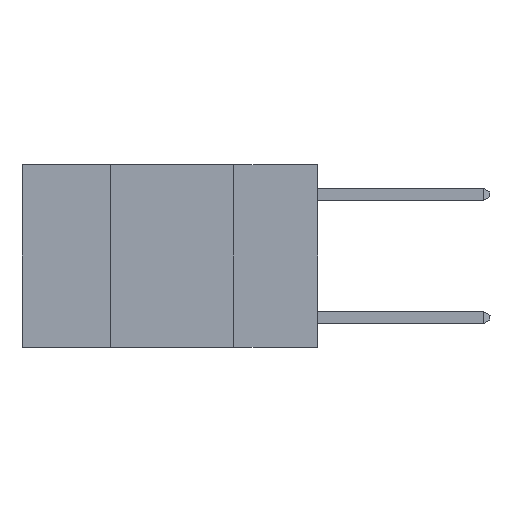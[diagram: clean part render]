
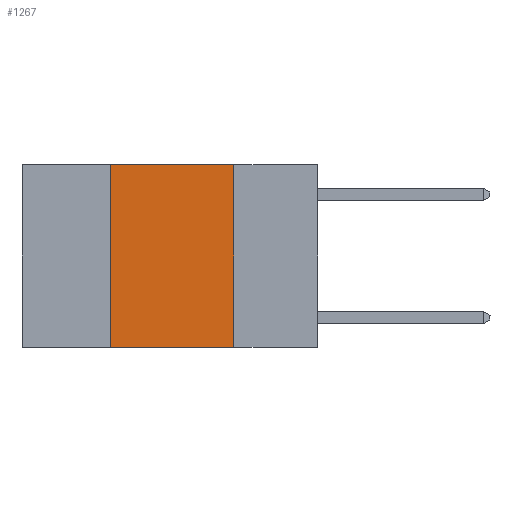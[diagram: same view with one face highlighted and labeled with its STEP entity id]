
A CAD part, left-side view. The second image highlights one B-rep face of the part: STEP entity #1267.
In plain terms, the highlighted planar face has unit normal (-1, 0, 0).
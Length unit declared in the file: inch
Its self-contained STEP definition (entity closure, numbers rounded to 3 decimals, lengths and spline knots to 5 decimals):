
#1013 = EDGE_CURVE ( 'NONE', #4432, #13708, #11321, .T. ) ;
#1029 = CARTESIAN_POINT ( 'NONE',  ( 0., 0.42, 0. ) ) ;
#1267 = ADVANCED_FACE ( 'NONE', ( #11890 ), #11979, .F. ) ;
#1552 = CARTESIAN_POINT ( 'NONE',  ( 0., 0.17, 0. ) ) ;
#1984 = VERTEX_POINT ( 'NONE', #16516 ) ;
#2218 = DIRECTION ( 'NONE',  ( 0., 0., 1. ) ) ;
#2761 = EDGE_CURVE ( 'NONE', #1984, #17518, #3835, .T. ) ;
#3797 = EDGE_CURVE ( 'NONE', #13708, #17518, #4165, .T. ) ;
#3835 = LINE ( 'NONE', #9848, #17311 ) ;
#4017 = CARTESIAN_POINT ( 'NONE',  ( 0., 0.6, 0. ) ) ;
#4165 = LINE ( 'NONE', #1552, #17338 ) ;
#4432 = VERTEX_POINT ( 'NONE', #6509 ) ;
#4508 = VECTOR ( 'NONE', #14210, 39.37008 ) ;
#5514 = EDGE_CURVE ( 'NONE', #1984, #4432, #8598, .T. ) ;
#6509 = CARTESIAN_POINT ( 'NONE',  ( 0., 0.42, 0. ) ) ;
#7921 = CARTESIAN_POINT ( 'NONE',  ( 0., 0.17, 0. ) ) ;
#8598 = LINE ( 'NONE', #1029, #18716 ) ;
#8946 = ORIENTED_EDGE ( 'NONE', *, *, #2761, .T. ) ;
#9848 = CARTESIAN_POINT ( 'NONE',  ( 0., 0.6, -0.37 ) ) ;
#10430 = DIRECTION ( 'NONE',  ( 0., 0., -1. ) ) ;
#11273 = ORIENTED_EDGE ( 'NONE', *, *, #5514, .F. ) ;
#11321 = LINE ( 'NONE', #4017, #4508 ) ;
#11365 = CARTESIAN_POINT ( 'NONE',  ( 0., 0.17, -0.37 ) ) ;
#11433 = AXIS2_PLACEMENT_3D ( 'NONE', #14890, #17794, #10430 ) ;
#11519 = DIRECTION ( 'NONE',  ( 0., -1., 0. ) ) ;
#11890 = FACE_OUTER_BOUND ( 'NONE', #14209, .T. ) ;
#11979 = PLANE ( 'NONE',  #11433 ) ;
#13494 = ORIENTED_EDGE ( 'NONE', *, *, #1013, .F. ) ;
#13708 = VERTEX_POINT ( 'NONE', #7921 ) ;
#14209 = EDGE_LOOP ( 'NONE', ( #15666, #13494, #11273, #8946 ) ) ;
#14210 = DIRECTION ( 'NONE',  ( 0., -1., 0. ) ) ;
#14890 = CARTESIAN_POINT ( 'NONE',  ( 0., 0.6, 0. ) ) ;
#14951 = DIRECTION ( 'NONE',  ( 0., 0., -1. ) ) ;
#15666 = ORIENTED_EDGE ( 'NONE', *, *, #3797, .F. ) ;
#16516 = CARTESIAN_POINT ( 'NONE',  ( 0., 0.42, -0.37 ) ) ;
#17311 = VECTOR ( 'NONE', #11519, 39.37008 ) ;
#17338 = VECTOR ( 'NONE', #14951, 39.37008 ) ;
#17518 = VERTEX_POINT ( 'NONE', #11365 ) ;
#17794 = DIRECTION ( 'NONE',  ( 1., 0., 0. ) ) ;
#18716 = VECTOR ( 'NONE', #2218, 39.37008 ) ;
